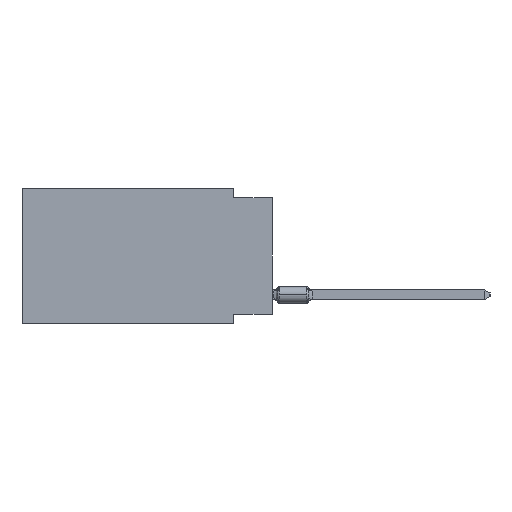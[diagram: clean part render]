
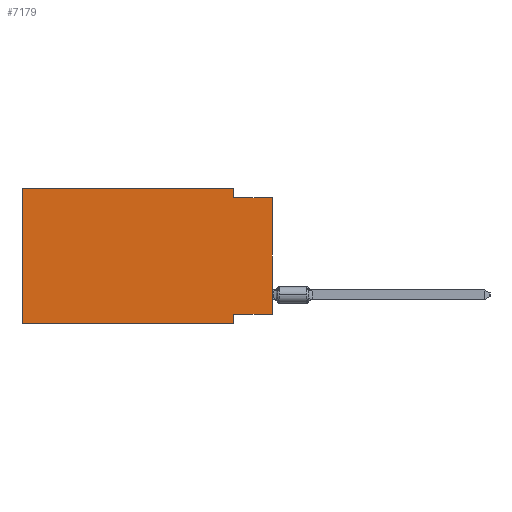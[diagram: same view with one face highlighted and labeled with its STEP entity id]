
A CAD part, left-side view. The second image highlights one B-rep face of the part: STEP entity #7179.
In plain terms, the highlighted planar face has unit normal (-1, 0, 0).
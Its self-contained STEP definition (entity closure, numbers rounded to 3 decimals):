
#401 = CARTESIAN_POINT ( 'NONE',  ( 0., 0., -8.255 ) ) ;
#1665 = VECTOR ( 'NONE', #36656, 1000. ) ;
#1821 = CARTESIAN_POINT ( 'NONE',  ( 0., 2.54, 0. ) ) ;
#4525 = VECTOR ( 'NONE', #30160, 1000. ) ;
#4847 = DIRECTION ( 'NONE',  ( 0., 0., 1. ) ) ;
#5099 = VERTEX_POINT ( 'NONE', #10978 ) ;
#6181 = EDGE_CURVE ( 'NONE', #23492, #16417, #20212, .T. ) ;
#6372 = EDGE_CURVE ( 'NONE', #28037, #35618, #27618, .T. ) ;
#6624 = CARTESIAN_POINT ( 'NONE',  ( 0., 16.383, -8.89 ) ) ;
#7043 = ORIENTED_EDGE ( 'NONE', *, *, #22108, .F. ) ;
#7179 = ADVANCED_FACE ( 'NONE', ( #38824 ), #39218, .F. ) ;
#7228 = EDGE_CURVE ( 'NONE', #35618, #37079, #33185, .T. ) ;
#7283 = VERTEX_POINT ( 'NONE', #6624 ) ;
#7853 = LINE ( 'NONE', #20101, #12106 ) ;
#9837 = LINE ( 'NONE', #21672, #39202 ) ;
#10387 = VECTOR ( 'NONE', #35183, 1000. ) ;
#10933 = ORIENTED_EDGE ( 'NONE', *, *, #30985, .F. ) ;
#10978 = CARTESIAN_POINT ( 'NONE',  ( 0., 0., -0.635 ) ) ;
#11034 = EDGE_CURVE ( 'NONE', #7283, #16417, #9837, .T. ) ;
#11259 = LINE ( 'NONE', #16883, #10387 ) ;
#11741 = ORIENTED_EDGE ( 'NONE', *, *, #14479, .T. ) ;
#11867 = DIRECTION ( 'NONE',  ( 1., 0., 0. ) ) ;
#12106 = VECTOR ( 'NONE', #4847, 1000. ) ;
#12353 = CARTESIAN_POINT ( 'NONE',  ( 0., 16.383, 0. ) ) ;
#14479 = EDGE_CURVE ( 'NONE', #25380, #5099, #11259, .T. ) ;
#15442 = DIRECTION ( 'NONE',  ( 0., -1., 0. ) ) ;
#16039 = DIRECTION ( 'NONE',  ( 0., 1., 0. ) ) ;
#16417 = VERTEX_POINT ( 'NONE', #38941 ) ;
#16883 = CARTESIAN_POINT ( 'NONE',  ( 0., 0., 0. ) ) ;
#17891 = CARTESIAN_POINT ( 'NONE',  ( 0., 2.54, 0. ) ) ;
#19853 = LINE ( 'NONE', #34551, #37787 ) ;
#19995 = CARTESIAN_POINT ( 'NONE',  ( 0., 2.54, -0.635 ) ) ;
#20101 = CARTESIAN_POINT ( 'NONE',  ( 0., 16.383, 0. ) ) ;
#20212 = LINE ( 'NONE', #35297, #35548 ) ;
#21360 = CARTESIAN_POINT ( 'NONE',  ( 0., 0., -0.635 ) ) ;
#21672 = CARTESIAN_POINT ( 'NONE',  ( 0., 16.383, -8.89 ) ) ;
#22108 = EDGE_CURVE ( 'NONE', #7283, #28037, #7853, .T. ) ;
#23492 = VERTEX_POINT ( 'NONE', #25495 ) ;
#24117 = CARTESIAN_POINT ( 'NONE',  ( 0., 16.383, 0. ) ) ;
#25380 = VERTEX_POINT ( 'NONE', #401 ) ;
#25495 = CARTESIAN_POINT ( 'NONE',  ( 0., 2.54, -8.255 ) ) ;
#26509 = EDGE_CURVE ( 'NONE', #37079, #5099, #27397, .T. ) ;
#27397 = LINE ( 'NONE', #21360, #1665 ) ;
#27618 = LINE ( 'NONE', #12353, #34248 ) ;
#28037 = VERTEX_POINT ( 'NONE', #35443 ) ;
#29392 = ORIENTED_EDGE ( 'NONE', *, *, #6181, .F. ) ;
#30160 = DIRECTION ( 'NONE',  ( 0., 0., -1. ) ) ;
#30859 = ORIENTED_EDGE ( 'NONE', *, *, #6372, .F. ) ;
#30985 = EDGE_CURVE ( 'NONE', #25380, #23492, #19853, .T. ) ;
#31313 = ORIENTED_EDGE ( 'NONE', *, *, #11034, .T. ) ;
#33185 = LINE ( 'NONE', #17891, #4525 ) ;
#33379 = DIRECTION ( 'NONE',  ( 0., 0., -1. ) ) ;
#33426 = AXIS2_PLACEMENT_3D ( 'NONE', #24117, #11867, #33379 ) ;
#33744 = ORIENTED_EDGE ( 'NONE', *, *, #7228, .F. ) ;
#34187 = EDGE_LOOP ( 'NONE', ( #11741, #34518, #33744, #30859, #7043, #31313, #29392, #10933 ) ) ;
#34248 = VECTOR ( 'NONE', #35901, 1000. ) ;
#34518 = ORIENTED_EDGE ( 'NONE', *, *, #26509, .F. ) ;
#34551 = CARTESIAN_POINT ( 'NONE',  ( 0., 0., -8.255 ) ) ;
#35183 = DIRECTION ( 'NONE',  ( 0., 0., 1. ) ) ;
#35297 = CARTESIAN_POINT ( 'NONE',  ( 0., 2.54, -8.89 ) ) ;
#35443 = CARTESIAN_POINT ( 'NONE',  ( 0., 16.383, 0. ) ) ;
#35548 = VECTOR ( 'NONE', #38709, 1000. ) ;
#35618 = VERTEX_POINT ( 'NONE', #1821 ) ;
#35901 = DIRECTION ( 'NONE',  ( 0., -1., 0. ) ) ;
#36656 = DIRECTION ( 'NONE',  ( 0., -1., 0. ) ) ;
#37079 = VERTEX_POINT ( 'NONE', #19995 ) ;
#37787 = VECTOR ( 'NONE', #16039, 1000. ) ;
#38709 = DIRECTION ( 'NONE',  ( 0., 0., -1. ) ) ;
#38824 = FACE_OUTER_BOUND ( 'NONE', #34187, .T. ) ;
#38941 = CARTESIAN_POINT ( 'NONE',  ( 0., 2.54, -8.89 ) ) ;
#39202 = VECTOR ( 'NONE', #15442, 1000. ) ;
#39218 = PLANE ( 'NONE',  #33426 ) ;
